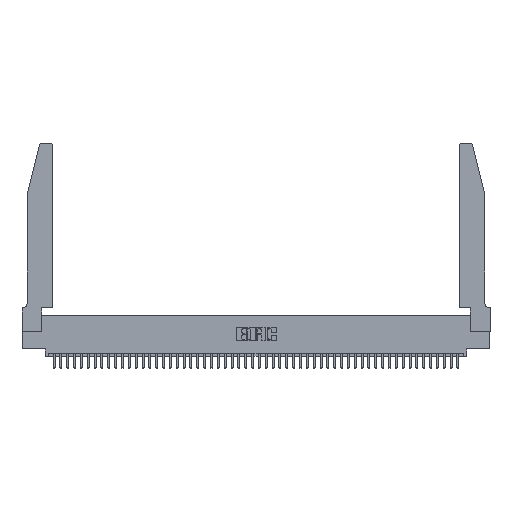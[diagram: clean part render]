
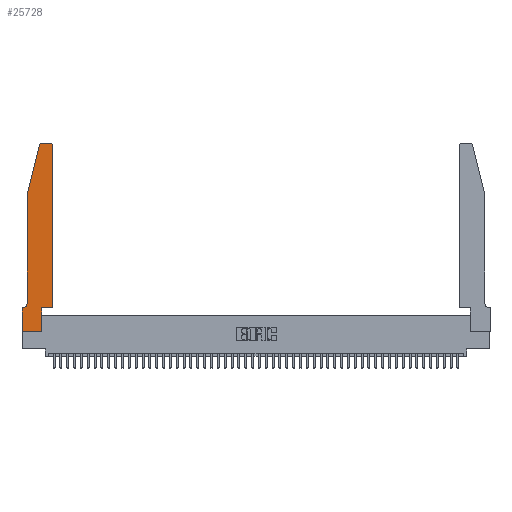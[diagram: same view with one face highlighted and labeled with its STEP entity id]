
A CAD part, top view. The second image highlights one B-rep face of the part: STEP entity #25728.
In plain terms, the highlighted planar face has unit normal (0, 0, 1).
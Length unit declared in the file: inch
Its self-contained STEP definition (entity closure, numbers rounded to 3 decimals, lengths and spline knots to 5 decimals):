
#862 = DIRECTION ( 'NONE',  ( 0., -1., 0. ) ) ;
#1034 = ORIENTED_EDGE ( 'NONE', *, *, #41272, .T. ) ;
#1091 = VERTEX_POINT ( 'NONE', #35152 ) ;
#1154 = EDGE_CURVE ( 'NONE', #1091, #28069, #5497, .T. ) ;
#1656 = CARTESIAN_POINT ( 'NONE',  ( 0.2865, 0.35, 0.37 ) ) ;
#3433 = DIRECTION ( 'NONE',  ( -1., 0., 0. ) ) ;
#3602 = DIRECTION ( 'NONE',  ( 1., 0., 0. ) ) ;
#3609 = VERTEX_POINT ( 'NONE', #13475 ) ;
#4011 = EDGE_CURVE ( 'NONE', #15614, #3609, #37039, .T. ) ;
#4684 = DIRECTION ( 'NONE',  ( 0., 1., 0. ) ) ;
#5247 = CARTESIAN_POINT ( 'NONE',  ( 0.2865, 0.35, 0.37 ) ) ;
#5497 = CIRCLE ( 'NONE', #21566, 0.03 ) ;
#7477 = ORIENTED_EDGE ( 'NONE', *, *, #15024, .T. ) ;
#7870 = CIRCLE ( 'NONE', #24014, 0.07 ) ;
#8528 = CARTESIAN_POINT ( 'NONE',  ( 0.25487, 2.72718, 0.37 ) ) ;
#9109 = CARTESIAN_POINT ( 'NONE',  ( 0.0755, 2., 0.37 ) ) ;
#10571 = ORIENTED_EDGE ( 'NONE', *, *, #24484, .T. ) ;
#10990 = CARTESIAN_POINT ( 'NONE',  ( 0.0755, 0.35, 0.37 ) ) ;
#11204 = EDGE_LOOP ( 'NONE', ( #10571, #1034, #40597, #41268, #44633, #39396, #48763, #17111, #14180, #16156, #7477, #13776 ) ) ;
#11338 = VECTOR ( 'NONE', #30506, 39.37008 ) ;
#11632 = VERTEX_POINT ( 'NONE', #45292 ) ;
#12491 = VECTOR ( 'NONE', #33989, 39.37008 ) ;
#13135 = EDGE_CURVE ( 'NONE', #17385, #15614, #26164, .T. ) ;
#13236 = AXIS2_PLACEMENT_3D ( 'NONE', #27178, #27506, #43060 ) ;
#13331 = CARTESIAN_POINT ( 'NONE',  ( 0., 0., 0.37 ) ) ;
#13475 = CARTESIAN_POINT ( 'NONE',  ( 0.4505, 0.35, 0.37 ) ) ;
#13776 = ORIENTED_EDGE ( 'NONE', *, *, #1154, .T. ) ;
#14180 = ORIENTED_EDGE ( 'NONE', *, *, #13135, .T. ) ;
#15024 = EDGE_CURVE ( 'NONE', #3609, #1091, #24236, .T. ) ;
#15614 = VERTEX_POINT ( 'NONE', #5247 ) ;
#16156 = ORIENTED_EDGE ( 'NONE', *, *, #4011, .T. ) ;
#16713 = CARTESIAN_POINT ( 'NONE',  ( 0.0055, 0.42, 0.37 ) ) ;
#17111 = ORIENTED_EDGE ( 'NONE', *, *, #46484, .T. ) ;
#17385 = VERTEX_POINT ( 'NONE', #19986 ) ;
#18151 = DIRECTION ( 'NONE',  ( 1., 0., 0. ) ) ;
#18156 = EDGE_CURVE ( 'NONE', #11632, #31015, #31732, .T. ) ;
#19051 = CARTESIAN_POINT ( 'NONE',  ( 0., 0., 0.37 ) ) ;
#19795 = CARTESIAN_POINT ( 'NONE',  ( 0.4505, 0.35, 0.37 ) ) ;
#19986 = CARTESIAN_POINT ( 'NONE',  ( 0.2865, 0., 0.37 ) ) ;
#20358 = CARTESIAN_POINT ( 'NONE',  ( 0.0055, 0.35, 0.37 ) ) ;
#21566 = AXIS2_PLACEMENT_3D ( 'NONE', #32273, #24870, #18151 ) ;
#22216 = CARTESIAN_POINT ( 'NONE',  ( 0., 0.35, 0.37 ) ) ;
#22381 = PLANE ( 'NONE',  #46516 ) ;
#22546 = DIRECTION ( 'NONE',  ( 0., 0., 1. ) ) ;
#22770 = LINE ( 'NONE', #9109, #48547 ) ;
#23313 = VERTEX_POINT ( 'NONE', #8528 ) ;
#23553 = VERTEX_POINT ( 'NONE', #44705 ) ;
#23660 = DIRECTION ( 'NONE',  ( 1., 0., 0. ) ) ;
#24014 = AXIS2_PLACEMENT_3D ( 'NONE', #16713, #28331, #40038 ) ;
#24236 = LINE ( 'NONE', #46771, #40438 ) ;
#24484 = EDGE_CURVE ( 'NONE', #28069, #23553, #39864, .T. ) ;
#24870 = DIRECTION ( 'NONE',  ( 0., 0., 1. ) ) ;
#24942 = VECTOR ( 'NONE', #47265, 39.37008 ) ;
#25728 = ADVANCED_FACE ( 'NONE', ( #31807 ), #22381, .T. ) ;
#26164 = LINE ( 'NONE', #1656, #24942 ) ;
#26575 = CARTESIAN_POINT ( 'NONE',  ( 0., 0., 0.37 ) ) ;
#26673 = VERTEX_POINT ( 'NONE', #44592 ) ;
#27178 = CARTESIAN_POINT ( 'NONE',  ( 0.284, 2.72, 0.37 ) ) ;
#27229 = CARTESIAN_POINT ( 'NONE',  ( 0.4205, 2.75, 0.37 ) ) ;
#27506 = DIRECTION ( 'NONE',  ( 0., 0., 1. ) ) ;
#28069 = VERTEX_POINT ( 'NONE', #27229 ) ;
#28331 = DIRECTION ( 'NONE',  ( 0., 0., -1. ) ) ;
#29921 = CARTESIAN_POINT ( 'NONE',  ( 0.2605, 2.75, 0.37 ) ) ;
#30506 = DIRECTION ( 'NONE',  ( 1., 0., 0. ) ) ;
#31015 = VERTEX_POINT ( 'NONE', #13331 ) ;
#31564 = EDGE_CURVE ( 'NONE', #31602, #26673, #48113, .T. ) ;
#31602 = VERTEX_POINT ( 'NONE', #32240 ) ;
#31732 = LINE ( 'NONE', #26575, #12491 ) ;
#31807 = FACE_OUTER_BOUND ( 'NONE', #11204, .T. ) ;
#32240 = CARTESIAN_POINT ( 'NONE',  ( 0.0755, 2., 0.37 ) ) ;
#32273 = CARTESIAN_POINT ( 'NONE',  ( 0.4205, 2.72, 0.37 ) ) ;
#33989 = DIRECTION ( 'NONE',  ( 0., -1., 0. ) ) ;
#34680 = VECTOR ( 'NONE', #3433, 39.37008 ) ;
#35152 = CARTESIAN_POINT ( 'NONE',  ( 0.4505, 2.72, 0.37 ) ) ;
#35762 = CARTESIAN_POINT ( 'NONE',  ( 0.0755, 2., 0.37 ) ) ;
#35845 = VECTOR ( 'NONE', #23660, 39.37008 ) ;
#35985 = LINE ( 'NONE', #19051, #11338 ) ;
#36017 = VERTEX_POINT ( 'NONE', #20358 ) ;
#36596 = EDGE_CURVE ( 'NONE', #26673, #36017, #7870, .T. ) ;
#37039 = LINE ( 'NONE', #19795, #35845 ) ;
#37041 = LINE ( 'NONE', #10990, #34680 ) ;
#37629 = EDGE_CURVE ( 'NONE', #23313, #31602, #22770, .T. ) ;
#37943 = VECTOR ( 'NONE', #862, 39.37008 ) ;
#39396 = ORIENTED_EDGE ( 'NONE', *, *, #43976, .T. ) ;
#39864 = LINE ( 'NONE', #29921, #42858 ) ;
#40038 = DIRECTION ( 'NONE',  ( -1., 0., 0. ) ) ;
#40438 = VECTOR ( 'NONE', #4684, 39.37008 ) ;
#40597 = ORIENTED_EDGE ( 'NONE', *, *, #37629, .T. ) ;
#41119 = DIRECTION ( 'NONE',  ( -1., 0., 0. ) ) ;
#41268 = ORIENTED_EDGE ( 'NONE', *, *, #31564, .T. ) ;
#41272 = EDGE_CURVE ( 'NONE', #23553, #23313, #48665, .T. ) ;
#42858 = VECTOR ( 'NONE', #41119, 39.37008 ) ;
#43060 = DIRECTION ( 'NONE',  ( 1., 0., 0. ) ) ;
#43976 = EDGE_CURVE ( 'NONE', #36017, #11632, #37041, .T. ) ;
#44592 = CARTESIAN_POINT ( 'NONE',  ( 0.0755, 0.42, 0.37 ) ) ;
#44633 = ORIENTED_EDGE ( 'NONE', *, *, #36596, .T. ) ;
#44705 = CARTESIAN_POINT ( 'NONE',  ( 0.284, 2.75, 0.37 ) ) ;
#45292 = CARTESIAN_POINT ( 'NONE',  ( 0., 0.35, 0.37 ) ) ;
#46484 = EDGE_CURVE ( 'NONE', #31015, #17385, #35985, .T. ) ;
#46516 = AXIS2_PLACEMENT_3D ( 'NONE', #22216, #22546, #3602 ) ;
#46771 = CARTESIAN_POINT ( 'NONE',  ( 0.4505, 0.35, 0.37 ) ) ;
#47265 = DIRECTION ( 'NONE',  ( 0., 1., 0. ) ) ;
#47474 = DIRECTION ( 'NONE',  ( -0.239, -0.971, 0. ) ) ;
#48113 = LINE ( 'NONE', #35762, #37943 ) ;
#48547 = VECTOR ( 'NONE', #47474, 39.37008 ) ;
#48665 = CIRCLE ( 'NONE', #13236, 0.03 ) ;
#48763 = ORIENTED_EDGE ( 'NONE', *, *, #18156, .T. ) ;
